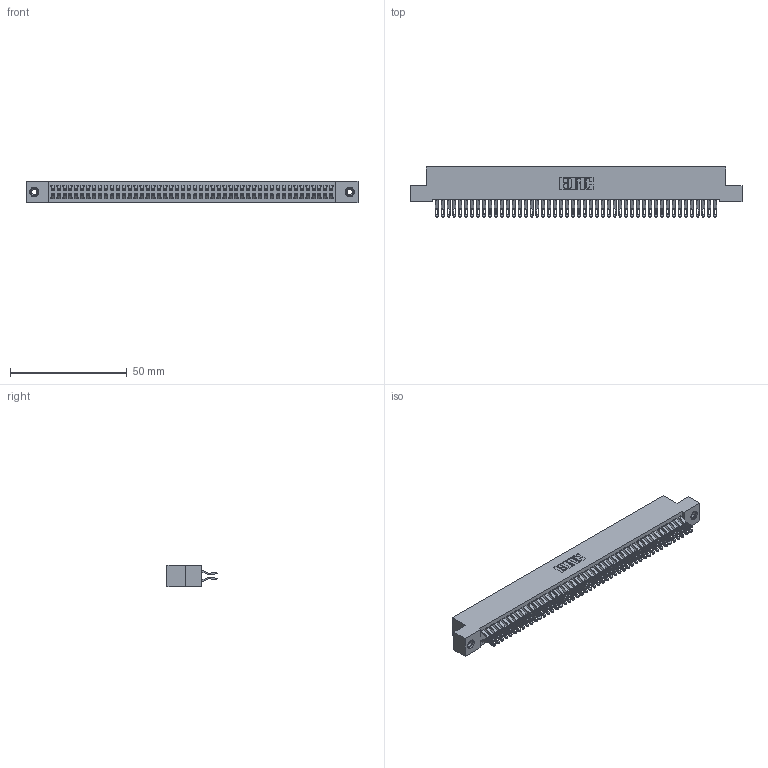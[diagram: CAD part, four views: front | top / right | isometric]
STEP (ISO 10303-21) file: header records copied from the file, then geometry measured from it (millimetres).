
FILE_DESCRIPTION (( 'STEP AP203' ), '1' );
FILE_NAME ('392-096-555-208.STEP', '2019-10-09T19:59:50', ( '' ), ( '' ), 'SwSTEP 2.0', 'SolidWorks 2016', '' );
FILE_SCHEMA (( 'CONFIG_CONTROL_DESIGN' ));
Length unit declared in the file: inch
Products named in the file (4): 345-292-001_555 Tail; 345-250-001_345-250-003-102; 392-096-555-208; 342 Part_TI
Assembly tree (99 placements, depth 2):
  392-096-555-208
    342 Part_TI
    345-292-001_555 Tail  x96
    345-250-001_345-250-003-102  x2
Bounding box: 142.24 x 21.47 x 9.4 mm (x, y, z)
Volume: 13069.7 mm3; surface area: 22361.2 mm2
Topology: 99 solids, 99 shells, 5738 faces, 18003 edges, 11994 vertices
Faces by surface type: plane 3362, cylinder 2360, cone 12, torus 4
Entity records: 31484 total; most frequent: CARTESIAN_POINT 5227, ORIENTED_EDGE 5126, DIRECTION 4457, EDGE_CURVE 2563, LINE 2395, VECTOR 2395, VERTEX_POINT 1704, AXIS2_PLACEMENT_3D 1031
